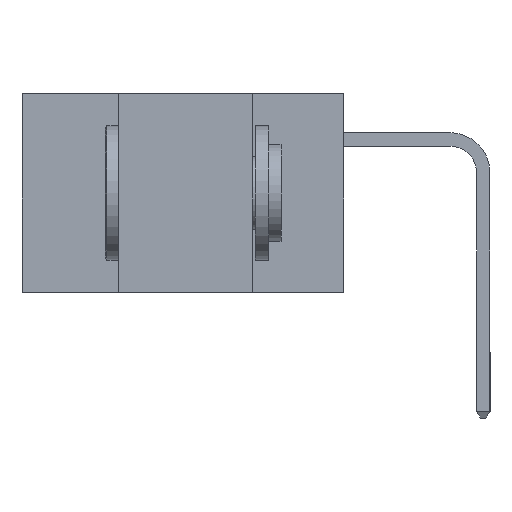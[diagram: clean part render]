
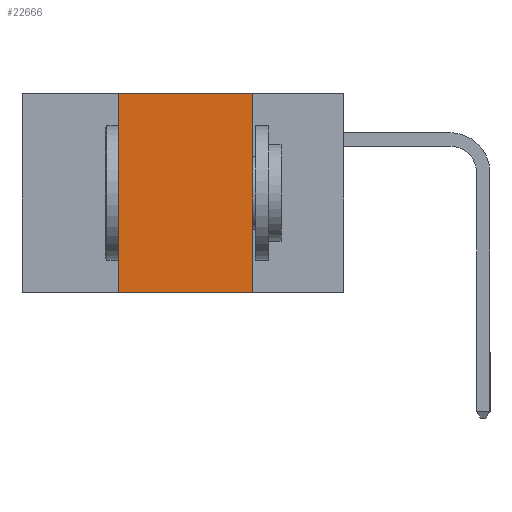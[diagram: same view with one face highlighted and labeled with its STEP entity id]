
A CAD part, left-side view. The second image highlights one B-rep face of the part: STEP entity #22666.
In plain terms, the highlighted planar face has unit normal (-1, 0, 0).
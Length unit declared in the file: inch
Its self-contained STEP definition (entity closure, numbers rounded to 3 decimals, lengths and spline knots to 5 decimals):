
#289 = VECTOR ( 'NONE', #10210, 39.37008 ) ;
#1771 = DIRECTION ( 'NONE',  ( 0., -1., 0. ) ) ;
#1971 = ORIENTED_EDGE ( 'NONE', *, *, #20468, .F. ) ;
#2520 = VECTOR ( 'NONE', #1771, 39.37008 ) ;
#3655 = EDGE_CURVE ( 'NONE', #21116, #25814, #6333, .T. ) ;
#3883 = VECTOR ( 'NONE', #11707, 39.37008 ) ;
#5777 = CARTESIAN_POINT ( 'NONE',  ( 0., 0.6, 0. ) ) ;
#6333 = LINE ( 'NONE', #11897, #3883 ) ;
#6965 = VERTEX_POINT ( 'NONE', #23080 ) ;
#7398 = CARTESIAN_POINT ( 'NONE',  ( 0., 0.6, 0. ) ) ;
#7599 = EDGE_CURVE ( 'NONE', #17286, #25814, #26658, .T. ) ;
#10210 = DIRECTION ( 'NONE',  ( 0., 0., 1. ) ) ;
#10266 = FACE_OUTER_BOUND ( 'NONE', #19487, .T. ) ;
#10876 = AXIS2_PLACEMENT_3D ( 'NONE', #7398, #25065, #11730 ) ;
#11707 = DIRECTION ( 'NONE',  ( 0., 0., -1. ) ) ;
#11730 = DIRECTION ( 'NONE',  ( 0., 0., -1. ) ) ;
#11897 = CARTESIAN_POINT ( 'NONE',  ( 0., 0.17, 0. ) ) ;
#12614 = ORIENTED_EDGE ( 'NONE', *, *, #7599, .T. ) ;
#13481 = VECTOR ( 'NONE', #17881, 39.37008 ) ;
#13813 = LINE ( 'NONE', #5777, #13481 ) ;
#14276 = LINE ( 'NONE', #21712, #289 ) ;
#16469 = CARTESIAN_POINT ( 'NONE',  ( 0., 0.17, 0. ) ) ;
#16855 = ORIENTED_EDGE ( 'NONE', *, *, #17495, .F. ) ;
#17286 = VERTEX_POINT ( 'NONE', #20836 ) ;
#17495 = EDGE_CURVE ( 'NONE', #6965, #21116, #13813, .T. ) ;
#17881 = DIRECTION ( 'NONE',  ( 0., -1., 0. ) ) ;
#18630 = PLANE ( 'NONE',  #10876 ) ;
#19487 = EDGE_LOOP ( 'NONE', ( #26563, #16855, #1971, #12614 ) ) ;
#20468 = EDGE_CURVE ( 'NONE', #17286, #6965, #14276, .T. ) ;
#20836 = CARTESIAN_POINT ( 'NONE',  ( 0., 0.42, -0.37 ) ) ;
#21116 = VERTEX_POINT ( 'NONE', #16469 ) ;
#21712 = CARTESIAN_POINT ( 'NONE',  ( 0., 0.42, 0. ) ) ;
#22666 = ADVANCED_FACE ( 'NONE', ( #10266 ), #18630, .F. ) ;
#23080 = CARTESIAN_POINT ( 'NONE',  ( 0., 0.42, 0. ) ) ;
#25065 = DIRECTION ( 'NONE',  ( 1., 0., 0. ) ) ;
#25814 = VERTEX_POINT ( 'NONE', #28862 ) ;
#25925 = CARTESIAN_POINT ( 'NONE',  ( 0., 0.6, -0.37 ) ) ;
#26563 = ORIENTED_EDGE ( 'NONE', *, *, #3655, .F. ) ;
#26658 = LINE ( 'NONE', #25925, #2520 ) ;
#28862 = CARTESIAN_POINT ( 'NONE',  ( 0., 0.17, -0.37 ) ) ;
